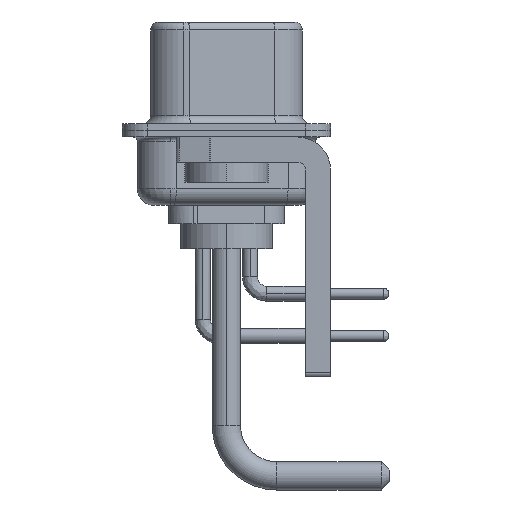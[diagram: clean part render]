
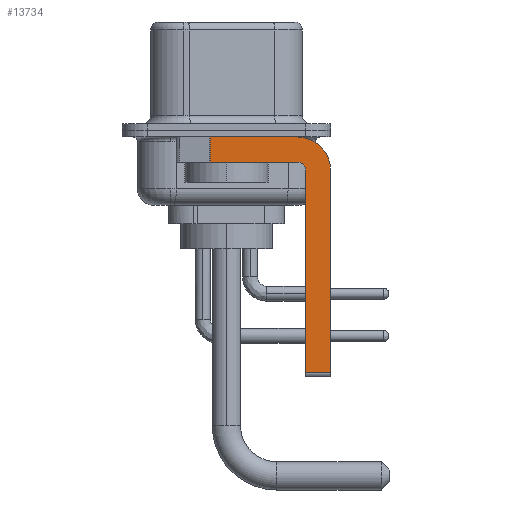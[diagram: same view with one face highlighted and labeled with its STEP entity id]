
A CAD part, left-side view. The second image highlights one B-rep face of the part: STEP entity #13734.
In plain terms, the highlighted planar face has unit normal (-1, 0, 0).
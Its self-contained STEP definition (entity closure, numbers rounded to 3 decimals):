
#22 = DIRECTION ( 'NONE',  ( 0., 0., -1. ) ) ;
#949 = CIRCLE ( 'NONE', #14756, 2. ) ;
#1889 = CARTESIAN_POINT ( 'NONE',  ( -2.9, 3., -0.4 ) ) ;
#2904 = DIRECTION ( 'NONE',  ( 0., 1., 0. ) ) ;
#4412 = CARTESIAN_POINT ( 'NONE',  ( -2.9, -4.75, -14.55 ) ) ;
#5112 = CARTESIAN_POINT ( 'NONE',  ( -2.9, -4.25, -2.4 ) ) ;
#5341 = CARTESIAN_POINT ( 'NONE',  ( -2.9, -4.25, -2.4 ) ) ;
#5546 = DIRECTION ( 'NONE',  ( 0., -1., 0. ) ) ;
#6031 = VERTEX_POINT ( 'NONE', #27361 ) ;
#6063 = VERTEX_POINT ( 'NONE', #4412 ) ;
#7430 = EDGE_CURVE ( 'NONE', #18300, #6031, #22680, .T. ) ;
#7541 = LINE ( 'NONE', #27821, #11598 ) ;
#7580 = LINE ( 'NONE', #10247, #19370 ) ;
#7925 = EDGE_CURVE ( 'NONE', #29328, #18300, #949, .T. ) ;
#8492 = DIRECTION ( 'NONE',  ( 1., 0., 0. ) ) ;
#8755 = LINE ( 'NONE', #13986, #20585 ) ;
#9941 = DIRECTION ( 'NONE',  ( 1., 0., 0. ) ) ;
#10049 = CARTESIAN_POINT ( 'NONE',  ( -2.9, -4.75, -2.4 ) ) ;
#10247 = CARTESIAN_POINT ( 'NONE',  ( -2.9, 0.978, -1.9 ) ) ;
#10309 = CARTESIAN_POINT ( 'NONE',  ( -2.9, 0.978, -1.9 ) ) ;
#11598 = VECTOR ( 'NONE', #2904, 1000. ) ;
#11777 = VECTOR ( 'NONE', #22, 1000. ) ;
#13412 = ORIENTED_EDGE ( 'NONE', *, *, #26161, .T. ) ;
#13734 = ADVANCED_FACE ( 'NONE', ( #21702 ), #18888, .F. ) ;
#13854 = DIRECTION ( 'NONE',  ( 0., 0., -1. ) ) ;
#13986 = CARTESIAN_POINT ( 'NONE',  ( -2.9, -4.75, -14.8 ) ) ;
#14756 = AXIS2_PLACEMENT_3D ( 'NONE', #19802, #8492, #13854 ) ;
#15709 = EDGE_CURVE ( 'NONE', #6063, #23590, #8755, .T. ) ;
#16151 = VECTOR ( 'NONE', #19775, 1000. ) ;
#16203 = AXIS2_PLACEMENT_3D ( 'NONE', #5341, #9941, #16817 ) ;
#16817 = DIRECTION ( 'NONE',  ( 0., 0., -1. ) ) ;
#17267 = LINE ( 'NONE', #1889, #16151 ) ;
#17361 = VECTOR ( 'NONE', #5546, 1000. ) ;
#17691 = VERTEX_POINT ( 'NONE', #21629 ) ;
#18300 = VERTEX_POINT ( 'NONE', #23061 ) ;
#18791 = ORIENTED_EDGE ( 'NONE', *, *, #23937, .F. ) ;
#18888 = PLANE ( 'NONE',  #16203 ) ;
#19370 = VECTOR ( 'NONE', #28581, 1000. ) ;
#19766 = CIRCLE ( 'NONE', #22653, 0.5 ) ;
#19775 = DIRECTION ( 'NONE',  ( 0., -1., 0. ) ) ;
#19802 = CARTESIAN_POINT ( 'NONE',  ( -2.9, -4.25, -2.4 ) ) ;
#20585 = VECTOR ( 'NONE', #25288, 1000. ) ;
#21181 = CARTESIAN_POINT ( 'NONE',  ( -2.9, -4.25, -14.55 ) ) ;
#21417 = VERTEX_POINT ( 'NONE', #22914 ) ;
#21450 = ORIENTED_EDGE ( 'NONE', *, *, #22681, .T. ) ;
#21629 = CARTESIAN_POINT ( 'NONE',  ( -2.9, 0.978, -0.4 ) ) ;
#21702 = FACE_OUTER_BOUND ( 'NONE', #28744, .T. ) ;
#22068 = EDGE_CURVE ( 'NONE', #21417, #24024, #7541, .T. ) ;
#22653 = AXIS2_PLACEMENT_3D ( 'NONE', #5112, #22842, #25659 ) ;
#22680 = LINE ( 'NONE', #28952, #11777 ) ;
#22681 = EDGE_CURVE ( 'NONE', #6063, #6031, #23856, .T. ) ;
#22842 = DIRECTION ( 'NONE',  ( -1., 0., 0. ) ) ;
#22914 = CARTESIAN_POINT ( 'NONE',  ( -2.9, -4.25, -1.9 ) ) ;
#23061 = CARTESIAN_POINT ( 'NONE',  ( -2.9, -6.25, -2.4 ) ) ;
#23590 = VERTEX_POINT ( 'NONE', #10049 ) ;
#23856 = LINE ( 'NONE', #21181, #17361 ) ;
#23935 = CARTESIAN_POINT ( 'NONE',  ( -2.9, -4.25, -0.4 ) ) ;
#23937 = EDGE_CURVE ( 'NONE', #23590, #21417, #19766, .T. ) ;
#24024 = VERTEX_POINT ( 'NONE', #10309 ) ;
#24125 = ORIENTED_EDGE ( 'NONE', *, *, #28848, .F. ) ;
#24423 = ORIENTED_EDGE ( 'NONE', *, *, #7925, .F. ) ;
#25288 = DIRECTION ( 'NONE',  ( 0., 0., 1. ) ) ;
#25659 = DIRECTION ( 'NONE',  ( 0., 0., 1. ) ) ;
#26161 = EDGE_CURVE ( 'NONE', #17691, #24024, #7580, .T. ) ;
#27361 = CARTESIAN_POINT ( 'NONE',  ( -2.9, -6.25, -14.55 ) ) ;
#27522 = ORIENTED_EDGE ( 'NONE', *, *, #22068, .F. ) ;
#27821 = CARTESIAN_POINT ( 'NONE',  ( -2.9, -4.25, -1.9 ) ) ;
#28581 = DIRECTION ( 'NONE',  ( 0., 0., -1. ) ) ;
#28744 = EDGE_LOOP ( 'NONE', ( #24125, #13412, #27522, #18791, #29023, #21450, #28771, #24423 ) ) ;
#28771 = ORIENTED_EDGE ( 'NONE', *, *, #7430, .F. ) ;
#28848 = EDGE_CURVE ( 'NONE', #17691, #29328, #17267, .T. ) ;
#28952 = CARTESIAN_POINT ( 'NONE',  ( -2.9, -6.25, -2.4 ) ) ;
#29023 = ORIENTED_EDGE ( 'NONE', *, *, #15709, .F. ) ;
#29328 = VERTEX_POINT ( 'NONE', #23935 ) ;
